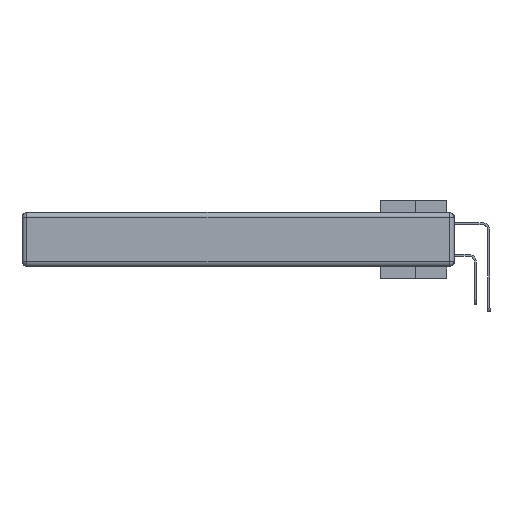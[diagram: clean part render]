
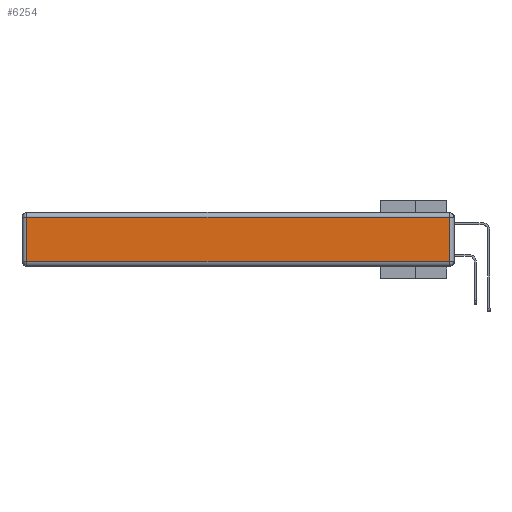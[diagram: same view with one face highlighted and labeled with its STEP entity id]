
A CAD part, left-side view. The second image highlights one B-rep face of the part: STEP entity #6254.
In plain terms, the highlighted planar face has unit normal (-1, 0, 0).
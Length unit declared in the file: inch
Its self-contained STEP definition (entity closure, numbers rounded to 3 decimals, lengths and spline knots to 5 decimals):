
#1746 = ORIENTED_EDGE ( 'NONE', *, *, #2103, .T. ) ;
#2103 = EDGE_CURVE ( 'NONE', #31948, #10006, #21514, .T. ) ;
#2348 = EDGE_CURVE ( 'NONE', #23528, #28259, #36377, .T. ) ;
#4332 = DIRECTION ( 'NONE',  ( -1., 0., 0. ) ) ;
#4770 = VECTOR ( 'NONE', #32966, 39.37008 ) ;
#5283 = VECTOR ( 'NONE', #30242, 39.37008 ) ;
#5706 = CARTESIAN_POINT ( 'NONE',  ( 0., 0., -0.313 ) ) ;
#5820 = VECTOR ( 'NONE', #15106, 39.37008 ) ;
#6254 = ADVANCED_FACE ( 'NONE', ( #12896 ), #22052, .T. ) ;
#6383 = DIRECTION ( 'NONE',  ( 0., 0., 1. ) ) ;
#7680 = CARTESIAN_POINT ( 'NONE',  ( 0., 2.72, -0.313 ) ) ;
#8748 = CARTESIAN_POINT ( 'NONE',  ( 0., 2.72, -0.343 ) ) ;
#8954 = ORIENTED_EDGE ( 'NONE', *, *, #2348, .T. ) ;
#10006 = VERTEX_POINT ( 'NONE', #34839 ) ;
#12896 = FACE_OUTER_BOUND ( 'NONE', #21142, .T. ) ;
#13878 = CARTESIAN_POINT ( 'NONE',  ( 0., 0., -0.343 ) ) ;
#14918 = CARTESIAN_POINT ( 'NONE',  ( 0., 0.03, -0.313 ) ) ;
#15106 = DIRECTION ( 'NONE',  ( 0., 0., -1. ) ) ;
#15119 = LINE ( 'NONE', #23891, #5283 ) ;
#17858 = VECTOR ( 'NONE', #6383, 39.37008 ) ;
#19455 = DIRECTION ( 'NONE',  ( 0., 0., 1. ) ) ;
#21142 = EDGE_LOOP ( 'NONE', ( #33167, #1746, #30999, #8954 ) ) ;
#21514 = LINE ( 'NONE', #33637, #17858 ) ;
#22052 = PLANE ( 'NONE',  #29209 ) ;
#23528 = VERTEX_POINT ( 'NONE', #31448 ) ;
#23891 = CARTESIAN_POINT ( 'NONE',  ( 0., 2.75, -0.03 ) ) ;
#24188 = EDGE_CURVE ( 'NONE', #28259, #31948, #27376, .T. ) ;
#27376 = LINE ( 'NONE', #5706, #4770 ) ;
#28259 = VERTEX_POINT ( 'NONE', #7680 ) ;
#29209 = AXIS2_PLACEMENT_3D ( 'NONE', #13878, #4332, #19455 ) ;
#30242 = DIRECTION ( 'NONE',  ( 0., 1., 0. ) ) ;
#30999 = ORIENTED_EDGE ( 'NONE', *, *, #34396, .T. ) ;
#31448 = CARTESIAN_POINT ( 'NONE',  ( 0., 2.72, -0.03 ) ) ;
#31948 = VERTEX_POINT ( 'NONE', #14918 ) ;
#32966 = DIRECTION ( 'NONE',  ( 0., -1., 0. ) ) ;
#33167 = ORIENTED_EDGE ( 'NONE', *, *, #24188, .T. ) ;
#33637 = CARTESIAN_POINT ( 'NONE',  ( 0., 0.03, -0.343 ) ) ;
#34396 = EDGE_CURVE ( 'NONE', #10006, #23528, #15119, .T. ) ;
#34839 = CARTESIAN_POINT ( 'NONE',  ( 0., 0.03, -0.03 ) ) ;
#36377 = LINE ( 'NONE', #8748, #5820 ) ;
